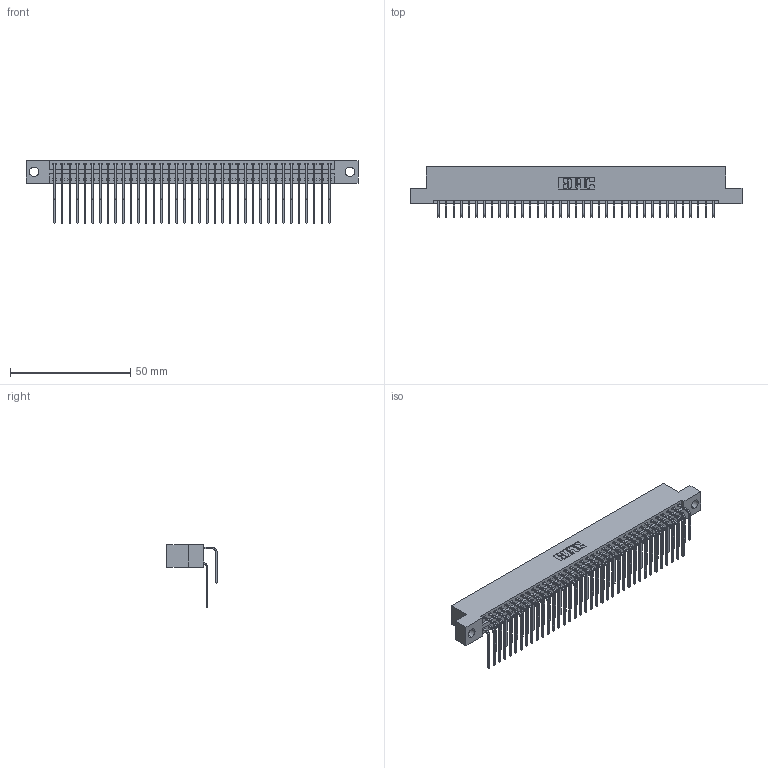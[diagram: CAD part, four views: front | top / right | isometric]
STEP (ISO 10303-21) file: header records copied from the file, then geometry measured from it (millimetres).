
FILE_DESCRIPTION (( 'STEP AP203' ), '1' );
FILE_NAME ('346-074-559-204.STEP', '2022-05-25T03:39:44', ( '' ), ( '' ), 'SwSTEP 2.0', 'SolidWorks 2020', '' );
FILE_SCHEMA (( 'CONFIG_CONTROL_DESIGN' ));
Length unit declared in the file: inch
Products named in the file (4): 346-074-559-204; 345-292-001_559 Tail - 2; 345-292-001_558 559 Tail - 1; 346 Part_Flush Mounting Lugs - 0.156 Dia-TH
Assembly tree (75 placements, depth 2):
  346-074-559-204
    346 Part_Flush Mounting Lugs - 0.156 Dia-TH
    345-292-001_558 559 Tail - 1  x37
    345-292-001_559 Tail - 2  x37
Bounding box: 138.05 x 20.89 x 26.16 mm (x, y, z)
Volume: 13743.6 mm3; surface area: 20708.7 mm2
Topology: 75 solids, 75 shells, 4132 faces, 12279 edges, 8086 vertices
Faces by surface type: plane 2828, cylinder 1304
Entity records: 27023 total; most frequent: CARTESIAN_POINT 4517, ORIENTED_EDGE 4398, DIRECTION 4003, EDGE_CURVE 2199, LINE 1879, VECTOR 1879, VERTEX_POINT 1462, AXIS2_PLACEMENT_3D 1062
